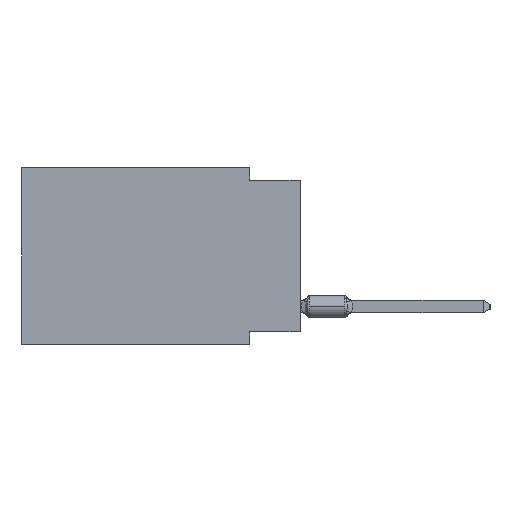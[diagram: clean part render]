
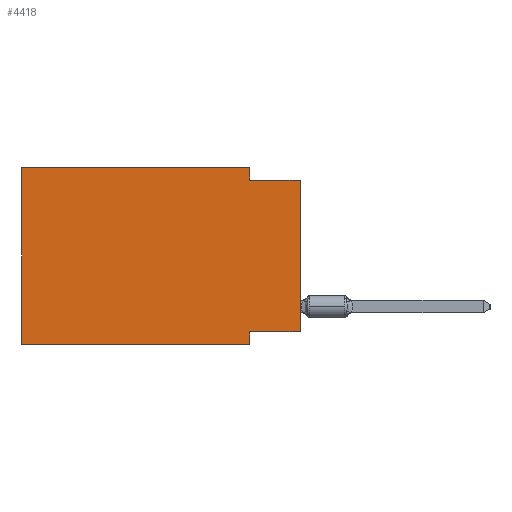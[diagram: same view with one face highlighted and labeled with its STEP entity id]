
A CAD part, left-side view. The second image highlights one B-rep face of the part: STEP entity #4418.
In plain terms, the highlighted planar face has unit normal (-1, 0, 0).
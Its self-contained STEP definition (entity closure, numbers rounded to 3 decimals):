
#567 = DIRECTION ( 'NONE',  ( 1., 0., 0. ) ) ;
#1489 = ORIENTED_EDGE ( 'NONE', *, *, #29213, .T. ) ;
#2909 = CARTESIAN_POINT ( 'NONE',  ( 0., 2.54, -8.89 ) ) ;
#4418 = ADVANCED_FACE ( 'NONE', ( #78622 ), #42699, .F. ) ;
#7545 = CARTESIAN_POINT ( 'NONE',  ( 0., 0., -8.255 ) ) ;
#8088 = LINE ( 'NONE', #36957, #84767 ) ;
#8130 = CARTESIAN_POINT ( 'NONE',  ( 0., 13.97, -8.89 ) ) ;
#14017 = EDGE_CURVE ( 'NONE', #19684, #53290, #15114, .T. ) ;
#15114 = LINE ( 'NONE', #7545, #75780 ) ;
#15192 = EDGE_CURVE ( 'NONE', #74488, #62429, #72811, .T. ) ;
#16702 = CARTESIAN_POINT ( 'NONE',  ( 0., 2.54, -8.255 ) ) ;
#18331 = VECTOR ( 'NONE', #47839, 1000. ) ;
#19684 = VERTEX_POINT ( 'NONE', #58405 ) ;
#21020 = DIRECTION ( 'NONE',  ( 0., -1., 0. ) ) ;
#22015 = EDGE_CURVE ( 'NONE', #30688, #80148, #8088, .T. ) ;
#25312 = EDGE_CURVE ( 'NONE', #19684, #54685, #61063, .T. ) ;
#29213 = EDGE_CURVE ( 'NONE', #74488, #90128, #40458, .T. ) ;
#30688 = VERTEX_POINT ( 'NONE', #76715 ) ;
#34913 = VECTOR ( 'NONE', #91950, 1000. ) ;
#35284 = ORIENTED_EDGE ( 'NONE', *, *, #61552, .F. ) ;
#35364 = EDGE_CURVE ( 'NONE', #80148, #54685, #40894, .T. ) ;
#36957 = CARTESIAN_POINT ( 'NONE',  ( 0., 2.54, 0. ) ) ;
#39341 = CARTESIAN_POINT ( 'NONE',  ( 0., 2.54, -0.635 ) ) ;
#40458 = LINE ( 'NONE', #84870, #74865 ) ;
#40894 = LINE ( 'NONE', #49392, #34913 ) ;
#42699 = PLANE ( 'NONE',  #78579 ) ;
#43159 = DIRECTION ( 'NONE',  ( 0., 0., -1. ) ) ;
#43614 = EDGE_CURVE ( 'NONE', #53290, #90128, #60635, .T. ) ;
#47839 = DIRECTION ( 'NONE',  ( 0., 0., -1. ) ) ;
#48305 = CARTESIAN_POINT ( 'NONE',  ( 0., 13.97, 0. ) ) ;
#49392 = CARTESIAN_POINT ( 'NONE',  ( 0., 0., -0.635 ) ) ;
#53290 = VERTEX_POINT ( 'NONE', #16702 ) ;
#54685 = VERTEX_POINT ( 'NONE', #62556 ) ;
#55407 = LINE ( 'NONE', #48305, #69146 ) ;
#56461 = CARTESIAN_POINT ( 'NONE',  ( 0., 13.97, 0. ) ) ;
#57360 = CARTESIAN_POINT ( 'NONE',  ( 0., 13.97, 0. ) ) ;
#57971 = ORIENTED_EDGE ( 'NONE', *, *, #25312, .T. ) ;
#58405 = CARTESIAN_POINT ( 'NONE',  ( 0., 0., -8.255 ) ) ;
#58719 = DIRECTION ( 'NONE',  ( 0., 0., -1. ) ) ;
#59643 = EDGE_LOOP ( 'NONE', ( #57971, #64372, #63017, #35284, #77480, #1489, #81915, #71035 ) ) ;
#60635 = LINE ( 'NONE', #2909, #18331 ) ;
#61063 = LINE ( 'NONE', #69078, #88686 ) ;
#61552 = EDGE_CURVE ( 'NONE', #62429, #30688, #55407, .T. ) ;
#61985 = DIRECTION ( 'NONE',  ( 0., 0., 1. ) ) ;
#62429 = VERTEX_POINT ( 'NONE', #56461 ) ;
#62556 = CARTESIAN_POINT ( 'NONE',  ( 0., 0., -0.635 ) ) ;
#63017 = ORIENTED_EDGE ( 'NONE', *, *, #22015, .F. ) ;
#64372 = ORIENTED_EDGE ( 'NONE', *, *, #35364, .F. ) ;
#67591 = DIRECTION ( 'NONE',  ( 0., 0., 1. ) ) ;
#68658 = DIRECTION ( 'NONE',  ( 0., -1., 0. ) ) ;
#69078 = CARTESIAN_POINT ( 'NONE',  ( 0., 0., 0. ) ) ;
#69146 = VECTOR ( 'NONE', #68658, 1000. ) ;
#71035 = ORIENTED_EDGE ( 'NONE', *, *, #14017, .F. ) ;
#72811 = LINE ( 'NONE', #79894, #81908 ) ;
#72817 = DIRECTION ( 'NONE',  ( 0., 1., 0. ) ) ;
#74488 = VERTEX_POINT ( 'NONE', #8130 ) ;
#74865 = VECTOR ( 'NONE', #21020, 1000. ) ;
#75780 = VECTOR ( 'NONE', #72817, 1000. ) ;
#76715 = CARTESIAN_POINT ( 'NONE',  ( 0., 2.54, 0. ) ) ;
#77480 = ORIENTED_EDGE ( 'NONE', *, *, #15192, .F. ) ;
#77596 = CARTESIAN_POINT ( 'NONE',  ( 0., 2.54, -8.89 ) ) ;
#78579 = AXIS2_PLACEMENT_3D ( 'NONE', #57360, #567, #43159 ) ;
#78622 = FACE_OUTER_BOUND ( 'NONE', #59643, .T. ) ;
#79894 = CARTESIAN_POINT ( 'NONE',  ( 0., 13.97, 0. ) ) ;
#80148 = VERTEX_POINT ( 'NONE', #39341 ) ;
#81908 = VECTOR ( 'NONE', #67591, 1000. ) ;
#81915 = ORIENTED_EDGE ( 'NONE', *, *, #43614, .F. ) ;
#84767 = VECTOR ( 'NONE', #58719, 1000. ) ;
#84870 = CARTESIAN_POINT ( 'NONE',  ( 0., 13.97, -8.89 ) ) ;
#88686 = VECTOR ( 'NONE', #61985, 1000. ) ;
#90128 = VERTEX_POINT ( 'NONE', #77596 ) ;
#91950 = DIRECTION ( 'NONE',  ( 0., -1., 0. ) ) ;
